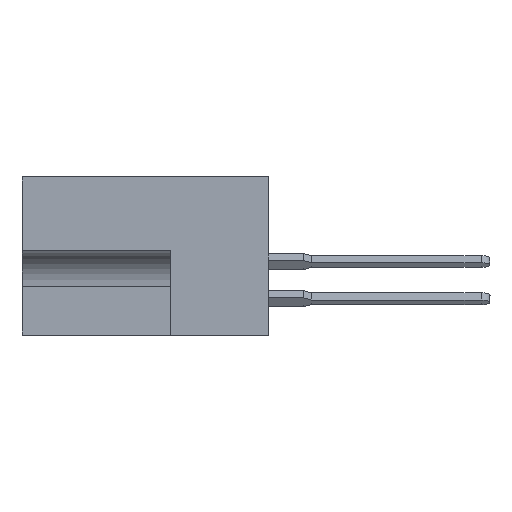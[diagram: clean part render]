
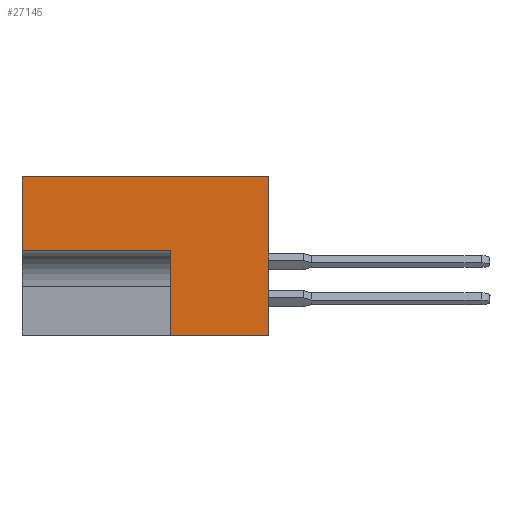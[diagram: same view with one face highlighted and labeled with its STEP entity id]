
A CAD part, left-side view. The second image highlights one B-rep face of the part: STEP entity #27145.
In plain terms, the highlighted planar face has unit normal (-1, 0, 0).
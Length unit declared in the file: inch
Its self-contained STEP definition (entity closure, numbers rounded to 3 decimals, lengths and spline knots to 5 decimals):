
#179 = LINE ( 'NONE', #251, #5337 ) ;
#251 = CARTESIAN_POINT ( 'NONE',  ( 0., 0.328, -0.531 ) ) ;
#1677 = LINE ( 'NONE', #10817, #21174 ) ;
#2245 = CARTESIAN_POINT ( 'NONE',  ( 0., 0., -0.531 ) ) ;
#2440 = VERTEX_POINT ( 'NONE', #3880 ) ;
#2583 = EDGE_LOOP ( 'NONE', ( #4970, #21997, #28697, #18821, #24392, #11093 ) ) ;
#3402 = DIRECTION ( 'NONE',  ( 0., 0., 1. ) ) ;
#3680 = EDGE_CURVE ( 'NONE', #29684, #12205, #17664, .T. ) ;
#3880 = CARTESIAN_POINT ( 'NONE',  ( 0., 0.828, -0.248 ) ) ;
#3911 = AXIS2_PLACEMENT_3D ( 'NONE', #8026, #19843, #26916 ) ;
#4286 = EDGE_CURVE ( 'NONE', #8287, #17566, #10233, .T. ) ;
#4687 = CARTESIAN_POINT ( 'NONE',  ( 0., 0.828, 0. ) ) ;
#4970 = ORIENTED_EDGE ( 'NONE', *, *, #11417, .F. ) ;
#5337 = VECTOR ( 'NONE', #11975, 39.37008 ) ;
#6148 = VECTOR ( 'NONE', #28667, 39.37008 ) ;
#7423 = VECTOR ( 'NONE', #3402, 39.37008 ) ;
#8026 = CARTESIAN_POINT ( 'NONE',  ( 0., 0.453, 0. ) ) ;
#8287 = VERTEX_POINT ( 'NONE', #12492 ) ;
#8291 = DIRECTION ( 'NONE',  ( 0., -1., 0. ) ) ;
#10233 = LINE ( 'NONE', #17514, #19055 ) ;
#10817 = CARTESIAN_POINT ( 'NONE',  ( 0., 0.828, 0. ) ) ;
#11093 = ORIENTED_EDGE ( 'NONE', *, *, #3680, .F. ) ;
#11163 = EDGE_CURVE ( 'NONE', #16011, #2440, #18279, .T. ) ;
#11417 = EDGE_CURVE ( 'NONE', #2440, #29684, #1677, .T. ) ;
#11975 = DIRECTION ( 'NONE',  ( 0., 0., 1. ) ) ;
#12205 = VERTEX_POINT ( 'NONE', #25845 ) ;
#12492 = CARTESIAN_POINT ( 'NONE',  ( 0., 0.328, -0.531 ) ) ;
#14837 = CARTESIAN_POINT ( 'NONE',  ( 0., 0.328, -0.248 ) ) ;
#15762 = DIRECTION ( 'NONE',  ( 0., 0., 1. ) ) ;
#16011 = VERTEX_POINT ( 'NONE', #19678 ) ;
#16624 = LINE ( 'NONE', #17399, #7423 ) ;
#17399 = CARTESIAN_POINT ( 'NONE',  ( 0., 0., 0. ) ) ;
#17514 = CARTESIAN_POINT ( 'NONE',  ( 0., 0.453, -0.531 ) ) ;
#17566 = VERTEX_POINT ( 'NONE', #2245 ) ;
#17664 = LINE ( 'NONE', #22182, #29481 ) ;
#18279 = LINE ( 'NONE', #14837, #6148 ) ;
#18821 = ORIENTED_EDGE ( 'NONE', *, *, #4286, .T. ) ;
#19055 = VECTOR ( 'NONE', #24529, 39.37008 ) ;
#19678 = CARTESIAN_POINT ( 'NONE',  ( 0., 0.328, -0.248 ) ) ;
#19738 = PLANE ( 'NONE',  #3911 ) ;
#19843 = DIRECTION ( 'NONE',  ( 1., 0., 0. ) ) ;
#21174 = VECTOR ( 'NONE', #15762, 39.37008 ) ;
#21997 = ORIENTED_EDGE ( 'NONE', *, *, #11163, .F. ) ;
#22182 = CARTESIAN_POINT ( 'NONE',  ( 0., 0.453, 0. ) ) ;
#24392 = ORIENTED_EDGE ( 'NONE', *, *, #27149, .T. ) ;
#24529 = DIRECTION ( 'NONE',  ( 0., -1., 0. ) ) ;
#24816 = EDGE_CURVE ( 'NONE', #8287, #16011, #179, .T. ) ;
#25845 = CARTESIAN_POINT ( 'NONE',  ( 0., 0., 0. ) ) ;
#26916 = DIRECTION ( 'NONE',  ( 0., 0., -1. ) ) ;
#27145 = ADVANCED_FACE ( 'NONE', ( #30297 ), #19738, .F. ) ;
#27149 = EDGE_CURVE ( 'NONE', #17566, #12205, #16624, .T. ) ;
#28667 = DIRECTION ( 'NONE',  ( 0., 1., 0. ) ) ;
#28697 = ORIENTED_EDGE ( 'NONE', *, *, #24816, .F. ) ;
#29481 = VECTOR ( 'NONE', #8291, 39.37008 ) ;
#29684 = VERTEX_POINT ( 'NONE', #4687 ) ;
#30297 = FACE_OUTER_BOUND ( 'NONE', #2583, .T. ) ;
